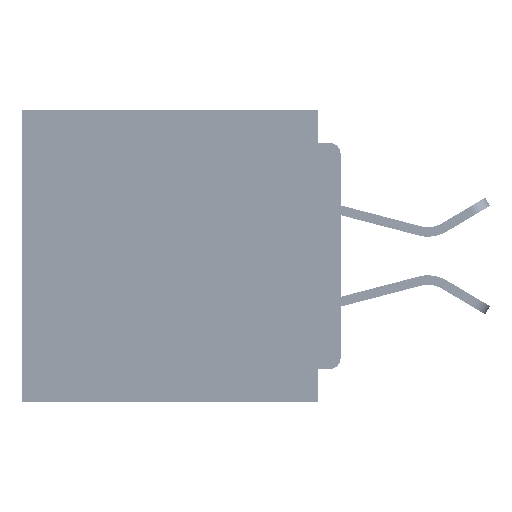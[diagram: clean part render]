
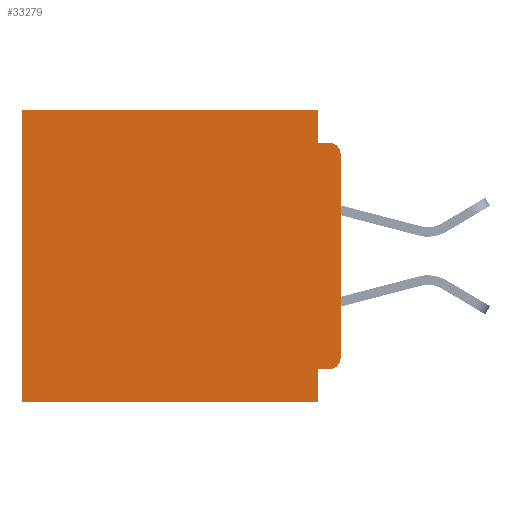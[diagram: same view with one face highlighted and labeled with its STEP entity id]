
A CAD part, left-side view. The second image highlights one B-rep face of the part: STEP entity #33279.
In plain terms, the highlighted planar face has unit normal (-1, 0, 0).
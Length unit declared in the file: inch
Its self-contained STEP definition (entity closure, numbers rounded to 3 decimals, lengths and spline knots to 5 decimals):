
#476 = AXIS2_PLACEMENT_3D ( 'NONE', #31230, #67756, #36545 ) ;
#602 = DIRECTION ( 'NONE',  ( -1., 0., 0. ) ) ;
#652 = EDGE_CURVE ( 'NONE', #22009, #11590, #63414, .T. ) ;
#1277 = ORIENTED_EDGE ( 'NONE', *, *, #57107, .F. ) ;
#1924 = VECTOR ( 'NONE', #66066, 39.37008 ) ;
#2101 = VECTOR ( 'NONE', #44677, 39.37008 ) ;
#5889 = LINE ( 'NONE', #22338, #18296 ) ;
#6280 = ORIENTED_EDGE ( 'NONE', *, *, #39255, .T. ) ;
#6504 = LINE ( 'NONE', #13661, #47029 ) ;
#7389 = VECTOR ( 'NONE', #50030, 39.37008 ) ;
#7870 = CARTESIAN_POINT ( 'NONE',  ( 0.3, 0.437, -0.4 ) ) ;
#8168 = CARTESIAN_POINT ( 'NONE',  ( 0.3, 0., -0.34 ) ) ;
#8246 = VERTEX_POINT ( 'NONE', #11957 ) ;
#8443 = VERTEX_POINT ( 'NONE', #45234 ) ;
#9226 = VERTEX_POINT ( 'NONE', #24836 ) ;
#10750 = DIRECTION ( 'NONE',  ( 1., 0., 0. ) ) ;
#11590 = VERTEX_POINT ( 'NONE', #59623 ) ;
#11683 = CARTESIAN_POINT ( 'NONE',  ( 0.3, 0.437, 0. ) ) ;
#11957 = CARTESIAN_POINT ( 'NONE',  ( 0.3, 0.031, 0. ) ) ;
#12174 = CARTESIAN_POINT ( 'NONE',  ( 0.3, 0.031, -0.355 ) ) ;
#13661 = CARTESIAN_POINT ( 'NONE',  ( 0.3, 0., -0.045 ) ) ;
#14015 = AXIS2_PLACEMENT_3D ( 'NONE', #32489, #602, #45629 ) ;
#14078 = ORIENTED_EDGE ( 'NONE', *, *, #40877, .F. ) ;
#16049 = LINE ( 'NONE', #61066, #1924 ) ;
#18296 = VECTOR ( 'NONE', #48614, 39.37008 ) ;
#19951 = EDGE_LOOP ( 'NONE', ( #43958, #52848, #1277, #14078, #65796, #6280, #45894, #38944, #63058, #52198 ) ) ;
#20540 = AXIS2_PLACEMENT_3D ( 'NONE', #42476, #10750, #47710 ) ;
#22009 = VERTEX_POINT ( 'NONE', #12174 ) ;
#22338 = CARTESIAN_POINT ( 'NONE',  ( 0.3, 0., 0. ) ) ;
#22867 = VERTEX_POINT ( 'NONE', #44440 ) ;
#23766 = EDGE_CURVE ( 'NONE', #9226, #34857, #35636, .T. ) ;
#24836 = CARTESIAN_POINT ( 'NONE',  ( 0.3, 0., -0.06 ) ) ;
#25273 = LINE ( 'NONE', #52535, #37712 ) ;
#26620 = DIRECTION ( 'NONE',  ( 0., 1., 0. ) ) ;
#26919 = VECTOR ( 'NONE', #61627, 39.37008 ) ;
#27292 = EDGE_CURVE ( 'NONE', #11590, #57892, #42606, .T. ) ;
#30389 = LINE ( 'NONE', #7870, #2101 ) ;
#30860 = VERTEX_POINT ( 'NONE', #8168 ) ;
#31230 = CARTESIAN_POINT ( 'NONE',  ( 0.3, 0.015, -0.06 ) ) ;
#32489 = CARTESIAN_POINT ( 'NONE',  ( 0.3, 0.015, -0.34 ) ) ;
#33279 = ADVANCED_FACE ( 'NONE', ( #37588 ), #63226, .F. ) ;
#34857 = VERTEX_POINT ( 'NONE', #40351 ) ;
#35636 = CIRCLE ( 'NONE', #476, 0.015 ) ;
#35874 = VERTEX_POINT ( 'NONE', #11683 ) ;
#36357 = CARTESIAN_POINT ( 'NONE',  ( 0.3, 0.437, -0.4 ) ) ;
#36545 = DIRECTION ( 'NONE',  ( 0., 0., -1. ) ) ;
#36907 = EDGE_CURVE ( 'NONE', #22867, #30860, #39003, .T. ) ;
#36962 = LINE ( 'NONE', #52762, #61451 ) ;
#37588 = FACE_OUTER_BOUND ( 'NONE', #19951, .T. ) ;
#37712 = VECTOR ( 'NONE', #57786, 39.37008 ) ;
#38944 = ORIENTED_EDGE ( 'NONE', *, *, #652, .F. ) ;
#39003 = CIRCLE ( 'NONE', #14015, 0.015 ) ;
#39255 = EDGE_CURVE ( 'NONE', #35874, #57892, #30389, .T. ) ;
#40351 = CARTESIAN_POINT ( 'NONE',  ( 0.3, 0.015, -0.045 ) ) ;
#40877 = EDGE_CURVE ( 'NONE', #8246, #8443, #25273, .T. ) ;
#42476 = CARTESIAN_POINT ( 'NONE',  ( 0.3, 0., -0.4 ) ) ;
#42606 = LINE ( 'NONE', #66841, #26919 ) ;
#43958 = ORIENTED_EDGE ( 'NONE', *, *, #67148, .F. ) ;
#44440 = CARTESIAN_POINT ( 'NONE',  ( 0.3, 0.015, -0.355 ) ) ;
#44677 = DIRECTION ( 'NONE',  ( 0., 0., -1. ) ) ;
#45234 = CARTESIAN_POINT ( 'NONE',  ( 0.3, 0.031, -0.045 ) ) ;
#45629 = DIRECTION ( 'NONE',  ( 0., 0., -1. ) ) ;
#45894 = ORIENTED_EDGE ( 'NONE', *, *, #27292, .F. ) ;
#47029 = VECTOR ( 'NONE', #55795, 39.37008 ) ;
#47710 = DIRECTION ( 'NONE',  ( 0., 0., -1. ) ) ;
#48614 = DIRECTION ( 'NONE',  ( 0., 1., 0. ) ) ;
#50030 = DIRECTION ( 'NONE',  ( 0., 0., -1. ) ) ;
#52198 = ORIENTED_EDGE ( 'NONE', *, *, #36907, .T. ) ;
#52535 = CARTESIAN_POINT ( 'NONE',  ( 0.3, 0.031, 0. ) ) ;
#52762 = CARTESIAN_POINT ( 'NONE',  ( 0.3, 0., -0.355 ) ) ;
#52848 = ORIENTED_EDGE ( 'NONE', *, *, #23766, .T. ) ;
#55795 = DIRECTION ( 'NONE',  ( 0., -1., 0. ) ) ;
#57107 = EDGE_CURVE ( 'NONE', #8443, #34857, #6504, .T. ) ;
#57786 = DIRECTION ( 'NONE',  ( 0., 0., -1. ) ) ;
#57892 = VERTEX_POINT ( 'NONE', #36357 ) ;
#59623 = CARTESIAN_POINT ( 'NONE',  ( 0.3, 0.031, -0.4 ) ) ;
#61066 = CARTESIAN_POINT ( 'NONE',  ( 0.3, 0., -0.4 ) ) ;
#61451 = VECTOR ( 'NONE', #26620, 39.37008 ) ;
#61627 = DIRECTION ( 'NONE',  ( 0., 1., 0. ) ) ;
#62063 = EDGE_CURVE ( 'NONE', #22867, #22009, #36962, .T. ) ;
#63058 = ORIENTED_EDGE ( 'NONE', *, *, #62063, .F. ) ;
#63226 = PLANE ( 'NONE',  #20540 ) ;
#63414 = LINE ( 'NONE', #63523, #7389 ) ;
#63523 = CARTESIAN_POINT ( 'NONE',  ( 0.3, 0.031, -0.4 ) ) ;
#65099 = EDGE_CURVE ( 'NONE', #8246, #35874, #5889, .T. ) ;
#65796 = ORIENTED_EDGE ( 'NONE', *, *, #65099, .T. ) ;
#66066 = DIRECTION ( 'NONE',  ( 0., 0., -1. ) ) ;
#66841 = CARTESIAN_POINT ( 'NONE',  ( 0.3, 0., -0.4 ) ) ;
#67148 = EDGE_CURVE ( 'NONE', #9226, #30860, #16049, .T. ) ;
#67756 = DIRECTION ( 'NONE',  ( -1., 0., 0. ) ) ;
